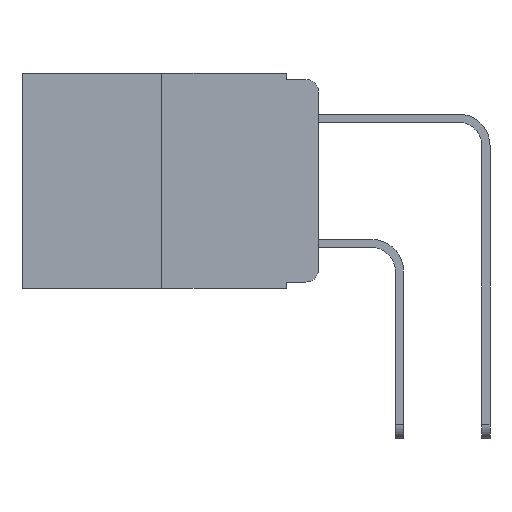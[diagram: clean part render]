
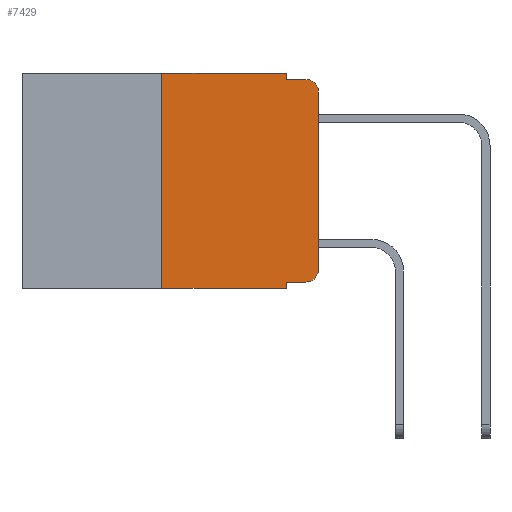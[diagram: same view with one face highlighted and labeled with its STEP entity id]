
A CAD part, left-side view. The second image highlights one B-rep face of the part: STEP entity #7429.
In plain terms, the highlighted planar face has unit normal (-1, 0, 0).
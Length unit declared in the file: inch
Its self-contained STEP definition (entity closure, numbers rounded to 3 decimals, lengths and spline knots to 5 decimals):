
#90 = DIRECTION ( 'NONE',  ( -1., 0., 0. ) ) ;
#700 = CIRCLE ( 'NONE', #7492, 0.02 ) ;
#1062 = VECTOR ( 'NONE', #4250, 39.37008 ) ;
#1187 = VERTEX_POINT ( 'NONE', #8207 ) ;
#1220 = EDGE_CURVE ( 'NONE', #5686, #1899, #6487, .T. ) ;
#1899 = VERTEX_POINT ( 'NONE', #13224 ) ;
#2028 = VERTEX_POINT ( 'NONE', #14205 ) ;
#2069 = AXIS2_PLACEMENT_3D ( 'NONE', #7605, #90, #8763 ) ;
#2195 = ORIENTED_EDGE ( 'NONE', *, *, #4881, .F. ) ;
#2331 = EDGE_CURVE ( 'NONE', #5634, #10753, #700, .T. ) ;
#2426 = ORIENTED_EDGE ( 'NONE', *, *, #14037, .T. ) ;
#2456 = ORIENTED_EDGE ( 'NONE', *, *, #4958, .F. ) ;
#2457 = ORIENTED_EDGE ( 'NONE', *, *, #5698, .F. ) ;
#2601 = VERTEX_POINT ( 'NONE', #6084 ) ;
#2675 = DIRECTION ( 'NONE',  ( 0., 0., -1. ) ) ;
#2754 = VECTOR ( 'NONE', #13119, 39.37008 ) ;
#2847 = ORIENTED_EDGE ( 'NONE', *, *, #3211, .T. ) ;
#3211 = EDGE_CURVE ( 'NONE', #7712, #5634, #13973, .T. ) ;
#3716 = VERTEX_POINT ( 'NONE', #14556 ) ;
#4058 = ORIENTED_EDGE ( 'NONE', *, *, #1220, .T. ) ;
#4116 = EDGE_CURVE ( 'NONE', #7712, #1899, #15057, .T. ) ;
#4250 = DIRECTION ( 'NONE',  ( 0., 0., 1. ) ) ;
#4881 = EDGE_CURVE ( 'NONE', #3716, #1187, #11939, .T. ) ;
#4954 = DIRECTION ( 'NONE',  ( 0., -1., 0. ) ) ;
#4958 = EDGE_CURVE ( 'NONE', #1187, #2028, #5415, .T. ) ;
#5034 = VECTOR ( 'NONE', #7631, 39.37008 ) ;
#5204 = VECTOR ( 'NONE', #9787, 39.37008 ) ;
#5279 = CARTESIAN_POINT ( 'NONE',  ( 0., 0.02, -0.333 ) ) ;
#5366 = CARTESIAN_POINT ( 'NONE',  ( 0., 0.25, -0.343 ) ) ;
#5415 = LINE ( 'NONE', #12843, #11025 ) ;
#5589 = VERTEX_POINT ( 'NONE', #12876 ) ;
#5634 = VERTEX_POINT ( 'NONE', #5279 ) ;
#5686 = VERTEX_POINT ( 'NONE', #5366 ) ;
#5698 = EDGE_CURVE ( 'NONE', #5686, #3716, #13468, .T. ) ;
#5891 = VECTOR ( 'NONE', #14457, 39.37008 ) ;
#6084 = CARTESIAN_POINT ( 'NONE',  ( 0., 0.02, -0.01 ) ) ;
#6093 = EDGE_LOOP ( 'NONE', ( #12366, #2426, #10610, #2456, #2195, #2457, #4058, #13352, #2847, #9518 ) ) ;
#6430 = CARTESIAN_POINT ( 'NONE',  ( 0., 0.473, -0.343 ) ) ;
#6460 = DIRECTION ( 'NONE',  ( 0., -1., 0. ) ) ;
#6487 = LINE ( 'NONE', #6430, #14813 ) ;
#6490 = EDGE_CURVE ( 'NONE', #2028, #2601, #8910, .T. ) ;
#6561 = CARTESIAN_POINT ( 'NONE',  ( 0., 0.051, 0. ) ) ;
#6827 = CARTESIAN_POINT ( 'NONE',  ( 0., 0.051, -0.01 ) ) ;
#6943 = CIRCLE ( 'NONE', #2069, 0.02 ) ;
#7391 = DIRECTION ( 'NONE',  ( 0., 0., -1. ) ) ;
#7429 = ADVANCED_FACE ( 'NONE', ( #11289 ), #12931, .F. ) ;
#7492 = AXIS2_PLACEMENT_3D ( 'NONE', #14470, #14356, #14372 ) ;
#7605 = CARTESIAN_POINT ( 'NONE',  ( 0., 0.02, -0.03 ) ) ;
#7631 = DIRECTION ( 'NONE',  ( 0., 0., 1. ) ) ;
#7712 = VERTEX_POINT ( 'NONE', #13374 ) ;
#8207 = CARTESIAN_POINT ( 'NONE',  ( 0., 0.051, 0. ) ) ;
#8763 = DIRECTION ( 'NONE',  ( 0., 0., -1. ) ) ;
#8910 = LINE ( 'NONE', #6827, #5891 ) ;
#9177 = CARTESIAN_POINT ( 'NONE',  ( 0., 0.051, -0.333 ) ) ;
#9518 = ORIENTED_EDGE ( 'NONE', *, *, #2331, .T. ) ;
#9558 = CARTESIAN_POINT ( 'NONE',  ( 0., 0., -0.313 ) ) ;
#9761 = DIRECTION ( 'NONE',  ( 1., 0., 0. ) ) ;
#9787 = DIRECTION ( 'NONE',  ( 0., -1., 0. ) ) ;
#9962 = CARTESIAN_POINT ( 'NONE',  ( 0., 0., 0. ) ) ;
#10610 = ORIENTED_EDGE ( 'NONE', *, *, #6490, .F. ) ;
#10753 = VERTEX_POINT ( 'NONE', #9558 ) ;
#11025 = VECTOR ( 'NONE', #7391, 39.37008 ) ;
#11289 = FACE_OUTER_BOUND ( 'NONE', #6093, .T. ) ;
#11939 = LINE ( 'NONE', #12716, #14730 ) ;
#12366 = ORIENTED_EDGE ( 'NONE', *, *, #13314, .T. ) ;
#12716 = CARTESIAN_POINT ( 'NONE',  ( 0., 0.473, 0. ) ) ;
#12843 = CARTESIAN_POINT ( 'NONE',  ( 0., 0.051, 0. ) ) ;
#12876 = CARTESIAN_POINT ( 'NONE',  ( 0., 0., -0.03 ) ) ;
#12931 = PLANE ( 'NONE',  #13560 ) ;
#13081 = CARTESIAN_POINT ( 'NONE',  ( 0., 0.25, 0. ) ) ;
#13119 = DIRECTION ( 'NONE',  ( 0., 0., -1. ) ) ;
#13224 = CARTESIAN_POINT ( 'NONE',  ( 0., 0.051, -0.343 ) ) ;
#13314 = EDGE_CURVE ( 'NONE', #10753, #5589, #13433, .T. ) ;
#13352 = ORIENTED_EDGE ( 'NONE', *, *, #4116, .F. ) ;
#13374 = CARTESIAN_POINT ( 'NONE',  ( 0., 0.051, -0.333 ) ) ;
#13433 = LINE ( 'NONE', #9962, #1062 ) ;
#13468 = LINE ( 'NONE', #13081, #5034 ) ;
#13560 = AXIS2_PLACEMENT_3D ( 'NONE', #13995, #9761, #2675 ) ;
#13973 = LINE ( 'NONE', #9177, #5204 ) ;
#13995 = CARTESIAN_POINT ( 'NONE',  ( 0., 0.473, 0. ) ) ;
#14037 = EDGE_CURVE ( 'NONE', #5589, #2601, #6943, .T. ) ;
#14205 = CARTESIAN_POINT ( 'NONE',  ( 0., 0.051, -0.01 ) ) ;
#14356 = DIRECTION ( 'NONE',  ( -1., 0., 0. ) ) ;
#14372 = DIRECTION ( 'NONE',  ( 0., 0., -1. ) ) ;
#14457 = DIRECTION ( 'NONE',  ( 0., -1., 0. ) ) ;
#14470 = CARTESIAN_POINT ( 'NONE',  ( 0., 0.02, -0.313 ) ) ;
#14556 = CARTESIAN_POINT ( 'NONE',  ( 0., 0.25, 0. ) ) ;
#14730 = VECTOR ( 'NONE', #4954, 39.37008 ) ;
#14813 = VECTOR ( 'NONE', #6460, 39.37008 ) ;
#15057 = LINE ( 'NONE', #6561, #2754 ) ;
